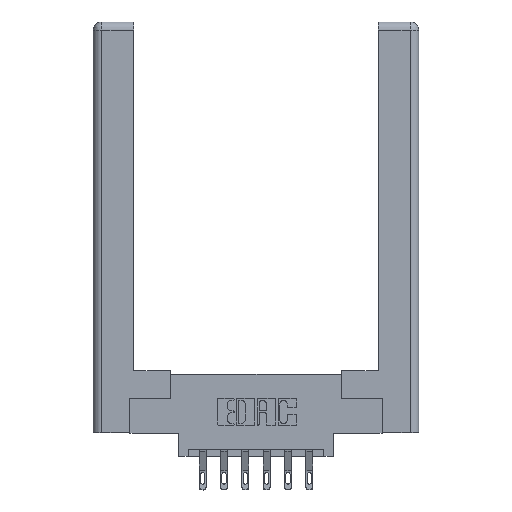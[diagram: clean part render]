
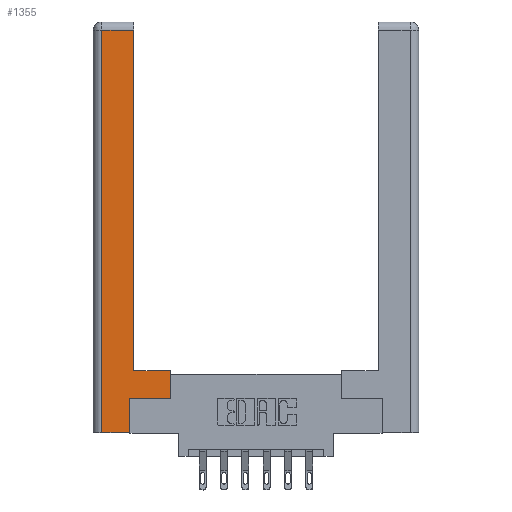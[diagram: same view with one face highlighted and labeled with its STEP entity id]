
A CAD part, top view. The second image highlights one B-rep face of the part: STEP entity #1355.
In plain terms, the highlighted planar face has unit normal (0, 0, 1).
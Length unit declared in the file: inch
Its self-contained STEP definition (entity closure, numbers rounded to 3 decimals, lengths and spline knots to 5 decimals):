
#206 = ORIENTED_EDGE ( 'NONE', *, *, #1196, .T. ) ;
#728 = CARTESIAN_POINT ( 'NONE',  ( 0.295, 2.94, 0. ) ) ;
#753 = DIRECTION ( 'NONE',  ( 0., 0., -1. ) ) ;
#898 = LINE ( 'NONE', #7644, #9339 ) ;
#907 = LINE ( 'NONE', #1430, #2271 ) ;
#1196 = EDGE_CURVE ( 'NONE', #11050, #8352, #907, .T. ) ;
#1295 = CARTESIAN_POINT ( 'NONE',  ( 0.0615, 2.94, 0. ) ) ;
#1308 = CARTESIAN_POINT ( 'NONE',  ( 0.295, 3., 0. ) ) ;
#1355 = ADVANCED_FACE ( 'NONE', ( #5572 ), #10946, .F. ) ;
#1373 = EDGE_CURVE ( 'NONE', #8352, #8801, #898, .T. ) ;
#1430 = CARTESIAN_POINT ( 'NONE',  ( 0.265, 0., 0. ) ) ;
#1788 = CARTESIAN_POINT ( 'NONE',  ( 0.565, 0.45, 0. ) ) ;
#2271 = VECTOR ( 'NONE', #10094, 39.37008 ) ;
#2704 = EDGE_CURVE ( 'NONE', #3767, #11050, #10937, .T. ) ;
#3254 = VECTOR ( 'NONE', #5256, 39.37008 ) ;
#3473 = DIRECTION ( 'NONE',  ( 1., 0., 0. ) ) ;
#3767 = VERTEX_POINT ( 'NONE', #5477 ) ;
#3787 = DIRECTION ( 'NONE',  ( -1., 0., 0. ) ) ;
#4126 = AXIS2_PLACEMENT_3D ( 'NONE', #5203, #753, #3787 ) ;
#4284 = EDGE_CURVE ( 'NONE', #11662, #6152, #5518, .T. ) ;
#4449 = DIRECTION ( 'NONE',  ( -1., 0., 0. ) ) ;
#4623 = CARTESIAN_POINT ( 'NONE',  ( 0.565, 0.245, 0. ) ) ;
#4844 = VERTEX_POINT ( 'NONE', #9588 ) ;
#5203 = CARTESIAN_POINT ( 'NONE',  ( 0., 0., 0. ) ) ;
#5256 = DIRECTION ( 'NONE',  ( 0., 1., 0. ) ) ;
#5371 = EDGE_CURVE ( 'NONE', #4844, #11662, #7478, .T. ) ;
#5477 = CARTESIAN_POINT ( 'NONE',  ( 0.0615, 2.94, 0. ) ) ;
#5518 = LINE ( 'NONE', #1308, #3254 ) ;
#5553 = DIRECTION ( 'NONE',  ( 0., 1., 0. ) ) ;
#5572 = FACE_OUTER_BOUND ( 'NONE', #5906, .T. ) ;
#5744 = ORIENTED_EDGE ( 'NONE', *, *, #9439, .T. ) ;
#5906 = EDGE_LOOP ( 'NONE', ( #10315, #11914, #9873, #206, #8878, #5744, #7387, #10034 ) ) ;
#6003 = CARTESIAN_POINT ( 'NONE',  ( 0.265, 0., 0. ) ) ;
#6152 = VERTEX_POINT ( 'NONE', #728 ) ;
#6656 = CARTESIAN_POINT ( 'NONE',  ( 0.0615, 0., 0. ) ) ;
#6666 = CARTESIAN_POINT ( 'NONE',  ( 0.295, 0.45, 0. ) ) ;
#7178 = VECTOR ( 'NONE', #10710, 39.37008 ) ;
#7387 = ORIENTED_EDGE ( 'NONE', *, *, #10843, .T. ) ;
#7403 = LINE ( 'NONE', #1295, #8458 ) ;
#7444 = VECTOR ( 'NONE', #12196, 39.37008 ) ;
#7478 = LINE ( 'NONE', #7809, #7178 ) ;
#7580 = DIRECTION ( 'NONE',  ( 0., -1., 0. ) ) ;
#7644 = CARTESIAN_POINT ( 'NONE',  ( 0.265, 0.245, 0. ) ) ;
#7809 = CARTESIAN_POINT ( 'NONE',  ( 0.295, 0.45, 0. ) ) ;
#8141 = VECTOR ( 'NONE', #7580, 39.37008 ) ;
#8211 = LINE ( 'NONE', #12071, #9230 ) ;
#8234 = CARTESIAN_POINT ( 'NONE',  ( 0.265, 0.245, 0. ) ) ;
#8352 = VERTEX_POINT ( 'NONE', #6003 ) ;
#8458 = VECTOR ( 'NONE', #4449, 39.37008 ) ;
#8801 = VERTEX_POINT ( 'NONE', #8234 ) ;
#8878 = ORIENTED_EDGE ( 'NONE', *, *, #1373, .T. ) ;
#9230 = VECTOR ( 'NONE', #3473, 39.37008 ) ;
#9339 = VECTOR ( 'NONE', #5553, 39.37008 ) ;
#9439 = EDGE_CURVE ( 'NONE', #8801, #10415, #8211, .T. ) ;
#9588 = CARTESIAN_POINT ( 'NONE',  ( 0.565, 0.45, 0. ) ) ;
#9873 = ORIENTED_EDGE ( 'NONE', *, *, #2704, .T. ) ;
#9977 = LINE ( 'NONE', #1788, #7444 ) ;
#10034 = ORIENTED_EDGE ( 'NONE', *, *, #5371, .T. ) ;
#10094 = DIRECTION ( 'NONE',  ( 1., 0., 0. ) ) ;
#10315 = ORIENTED_EDGE ( 'NONE', *, *, #4284, .T. ) ;
#10415 = VERTEX_POINT ( 'NONE', #4623 ) ;
#10710 = DIRECTION ( 'NONE',  ( -1., 0., 0. ) ) ;
#10843 = EDGE_CURVE ( 'NONE', #10415, #4844, #9977, .T. ) ;
#10937 = LINE ( 'NONE', #6656, #8141 ) ;
#10946 = PLANE ( 'NONE',  #4126 ) ;
#11050 = VERTEX_POINT ( 'NONE', #11765 ) ;
#11662 = VERTEX_POINT ( 'NONE', #6666 ) ;
#11765 = CARTESIAN_POINT ( 'NONE',  ( 0.0615, 0., 0. ) ) ;
#11914 = ORIENTED_EDGE ( 'NONE', *, *, #11979, .T. ) ;
#11979 = EDGE_CURVE ( 'NONE', #6152, #3767, #7403, .T. ) ;
#12071 = CARTESIAN_POINT ( 'NONE',  ( 0.565, 0.245, 0. ) ) ;
#12196 = DIRECTION ( 'NONE',  ( 0., 1., 0. ) ) ;
